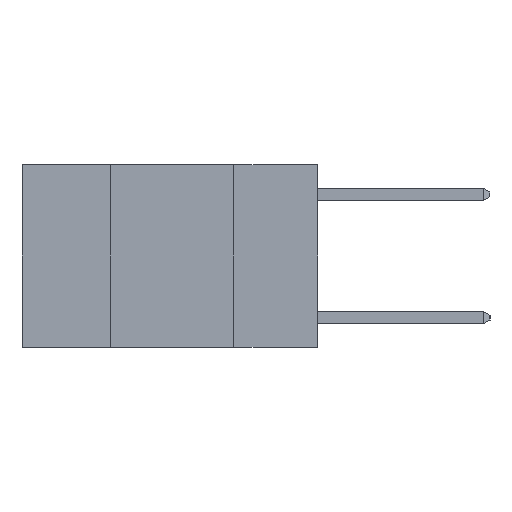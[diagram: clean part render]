
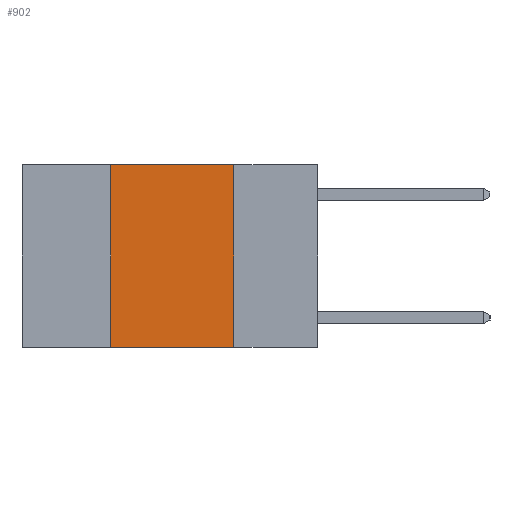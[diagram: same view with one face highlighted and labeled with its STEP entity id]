
A CAD part, left-side view. The second image highlights one B-rep face of the part: STEP entity #902.
In plain terms, the highlighted planar face has unit normal (-1, 0, 0).
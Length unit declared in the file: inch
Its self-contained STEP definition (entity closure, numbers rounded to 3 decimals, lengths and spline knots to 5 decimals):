
#94 = ORIENTED_EDGE ( 'NONE', *, *, #3704, .T. ) ;
#167 = VERTEX_POINT ( 'NONE', #8584 ) ;
#683 = FACE_OUTER_BOUND ( 'NONE', #4547, .T. ) ;
#755 = EDGE_CURVE ( 'NONE', #2317, #9300, #4501, .T. ) ;
#902 = ADVANCED_FACE ( 'NONE', ( #683 ), #9862, .F. ) ;
#1611 = LINE ( 'NONE', #8962, #5506 ) ;
#2317 = VERTEX_POINT ( 'NONE', #2839 ) ;
#2394 = CARTESIAN_POINT ( 'NONE',  ( 0., 0.17, 0. ) ) ;
#2688 = CARTESIAN_POINT ( 'NONE',  ( 0., 0.6, -0.37 ) ) ;
#2747 = DIRECTION ( 'NONE',  ( 0., 0., 1. ) ) ;
#2839 = CARTESIAN_POINT ( 'NONE',  ( 0., 0.42, -0.37 ) ) ;
#2994 = CARTESIAN_POINT ( 'NONE',  ( 0., 0.42, 0. ) ) ;
#3185 = VECTOR ( 'NONE', #4873, 39.37008 ) ;
#3191 = VECTOR ( 'NONE', #3487, 39.37008 ) ;
#3311 = EDGE_CURVE ( 'NONE', #5642, #167, #1611, .T. ) ;
#3487 = DIRECTION ( 'NONE',  ( 0., -1., 0. ) ) ;
#3704 = EDGE_CURVE ( 'NONE', #2317, #167, #7237, .T. ) ;
#4097 = CARTESIAN_POINT ( 'NONE',  ( 0., 0.6, 0. ) ) ;
#4252 = VECTOR ( 'NONE', #2747, 39.37008 ) ;
#4501 = LINE ( 'NONE', #2994, #4252 ) ;
#4547 = EDGE_LOOP ( 'NONE', ( #4999, #4806, #5944, #94 ) ) ;
#4806 = ORIENTED_EDGE ( 'NONE', *, *, #6434, .F. ) ;
#4873 = DIRECTION ( 'NONE',  ( 0., -1., 0. ) ) ;
#4999 = ORIENTED_EDGE ( 'NONE', *, *, #3311, .F. ) ;
#5506 = VECTOR ( 'NONE', #9733, 39.37008 ) ;
#5642 = VERTEX_POINT ( 'NONE', #2394 ) ;
#5944 = ORIENTED_EDGE ( 'NONE', *, *, #755, .F. ) ;
#6434 = EDGE_CURVE ( 'NONE', #9300, #5642, #7231, .T. ) ;
#7231 = LINE ( 'NONE', #4097, #3185 ) ;
#7237 = LINE ( 'NONE', #2688, #3191 ) ;
#7862 = CARTESIAN_POINT ( 'NONE',  ( 0., 0.42, 0. ) ) ;
#8584 = CARTESIAN_POINT ( 'NONE',  ( 0., 0.17, -0.37 ) ) ;
#8880 = AXIS2_PLACEMENT_3D ( 'NONE', #9925, #9833, #9831 ) ;
#8962 = CARTESIAN_POINT ( 'NONE',  ( 0., 0.17, 0. ) ) ;
#9300 = VERTEX_POINT ( 'NONE', #7862 ) ;
#9733 = DIRECTION ( 'NONE',  ( 0., 0., -1. ) ) ;
#9831 = DIRECTION ( 'NONE',  ( 0., 0., -1. ) ) ;
#9833 = DIRECTION ( 'NONE',  ( 1., 0., 0. ) ) ;
#9862 = PLANE ( 'NONE',  #8880 ) ;
#9925 = CARTESIAN_POINT ( 'NONE',  ( 0., 0.6, 0. ) ) ;
